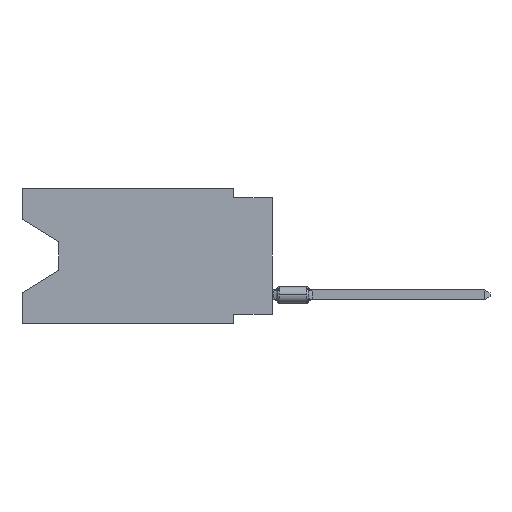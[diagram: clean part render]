
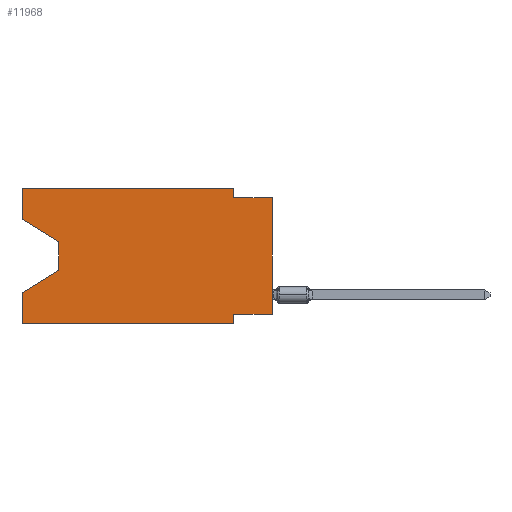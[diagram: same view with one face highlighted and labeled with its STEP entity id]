
A CAD part, left-side view. The second image highlights one B-rep face of the part: STEP entity #11968.
In plain terms, the highlighted planar face has unit normal (-1, 0, 0).
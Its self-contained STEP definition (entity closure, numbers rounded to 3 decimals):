
#106 = EDGE_CURVE ( 'NONE', #3288, #13067, #16867, .T. ) ;
#552 = CARTESIAN_POINT ( 'NONE',  ( 0., 2.54, 0. ) ) ;
#591 = DIRECTION ( 'NONE',  ( 0., 1., 0. ) ) ;
#726 = VECTOR ( 'NONE', #15065, 1000. ) ;
#868 = VECTOR ( 'NONE', #11107, 1000. ) ;
#931 = VECTOR ( 'NONE', #11445, 1000. ) ;
#1129 = CARTESIAN_POINT ( 'NONE',  ( 0., 16.383, -2.038 ) ) ;
#1162 = ORIENTED_EDGE ( 'NONE', *, *, #19828, .T. ) ;
#1165 = VERTEX_POINT ( 'NONE', #9282 ) ;
#1702 = VECTOR ( 'NONE', #10590, 1000. ) ;
#1963 = CARTESIAN_POINT ( 'NONE',  ( 0., 0., -0.635 ) ) ;
#2157 = VERTEX_POINT ( 'NONE', #18144 ) ;
#2304 = CARTESIAN_POINT ( 'NONE',  ( 0., 0., -8.255 ) ) ;
#2683 = VERTEX_POINT ( 'NONE', #5898 ) ;
#2824 = ORIENTED_EDGE ( 'NONE', *, *, #8476, .T. ) ;
#3091 = CARTESIAN_POINT ( 'NONE',  ( 0., 2.54, 0. ) ) ;
#3111 = PLANE ( 'NONE',  #18982 ) ;
#3288 = VERTEX_POINT ( 'NONE', #23810 ) ;
#3625 = CARTESIAN_POINT ( 'NONE',  ( 0., 0., -0.635 ) ) ;
#3835 = VECTOR ( 'NONE', #10383, 1000. ) ;
#3993 = VERTEX_POINT ( 'NONE', #21806 ) ;
#4361 = CARTESIAN_POINT ( 'NONE',  ( 0., 16.383, -8.89 ) ) ;
#5076 = DIRECTION ( 'NONE',  ( 1., 0., 0. ) ) ;
#5306 = EDGE_CURVE ( 'NONE', #2157, #2683, #7173, .T. ) ;
#5634 = ORIENTED_EDGE ( 'NONE', *, *, #13589, .F. ) ;
#5898 = CARTESIAN_POINT ( 'NONE',  ( 0., 2.54, -8.89 ) ) ;
#6046 = CARTESIAN_POINT ( 'NONE',  ( 0., 16.383, -2.038 ) ) ;
#6144 = EDGE_LOOP ( 'NONE', ( #1162, #20517, #16473, #9289, #6242, #10947, #17091, #2824, #5634, #23249, #10816, #18569 ) ) ;
#6242 = ORIENTED_EDGE ( 'NONE', *, *, #17470, .T. ) ;
#6563 = CARTESIAN_POINT ( 'NONE',  ( 0., 16.383, 0. ) ) ;
#6565 = EDGE_CURVE ( 'NONE', #3993, #3288, #13773, .T. ) ;
#6923 = CARTESIAN_POINT ( 'NONE',  ( 0., 16.383, 0. ) ) ;
#6986 = EDGE_CURVE ( 'NONE', #16297, #1165, #12475, .T. ) ;
#7022 = LINE ( 'NONE', #12564, #1702 ) ;
#7173 = LINE ( 'NONE', #12837, #11865 ) ;
#7303 = VERTEX_POINT ( 'NONE', #22535 ) ;
#7322 = LINE ( 'NONE', #13110, #726 ) ;
#7744 = LINE ( 'NONE', #1963, #931 ) ;
#8208 = EDGE_CURVE ( 'NONE', #11666, #19872, #11739, .T. ) ;
#8476 = EDGE_CURVE ( 'NONE', #7303, #21002, #22764, .T. ) ;
#9282 = CARTESIAN_POINT ( 'NONE',  ( 0., 16.383, 0. ) ) ;
#9289 = ORIENTED_EDGE ( 'NONE', *, *, #12259, .F. ) ;
#9373 = VERTEX_POINT ( 'NONE', #4361 ) ;
#10278 = EDGE_CURVE ( 'NONE', #7303, #2157, #11542, .T. ) ;
#10383 = DIRECTION ( 'NONE',  ( 0., 0., 1. ) ) ;
#10486 = LINE ( 'NONE', #1129, #12866 ) ;
#10590 = DIRECTION ( 'NONE',  ( 0., 0., 1. ) ) ;
#10816 = ORIENTED_EDGE ( 'NONE', *, *, #16095, .F. ) ;
#10947 = ORIENTED_EDGE ( 'NONE', *, *, #5306, .F. ) ;
#11107 = DIRECTION ( 'NONE',  ( 0., 0., 1. ) ) ;
#11354 = DIRECTION ( 'NONE',  ( 0., 0., -1. ) ) ;
#11445 = DIRECTION ( 'NONE',  ( 0., -1., 0. ) ) ;
#11542 = LINE ( 'NONE', #2304, #17362 ) ;
#11579 = CARTESIAN_POINT ( 'NONE',  ( 0., 13.97, -5.385 ) ) ;
#11666 = VERTEX_POINT ( 'NONE', #3091 ) ;
#11739 = LINE ( 'NONE', #552, #18933 ) ;
#11865 = VECTOR ( 'NONE', #11354, 1000. ) ;
#11869 = DIRECTION ( 'NONE',  ( 0., 0., -1. ) ) ;
#11968 = ADVANCED_FACE ( 'NONE', ( #21800 ), #3111, .F. ) ;
#12259 = EDGE_CURVE ( 'NONE', #9373, #13067, #7022, .T. ) ;
#12470 = LINE ( 'NONE', #19954, #19007 ) ;
#12475 = LINE ( 'NONE', #6563, #3835 ) ;
#12564 = CARTESIAN_POINT ( 'NONE',  ( 0., 16.383, 0. ) ) ;
#12837 = CARTESIAN_POINT ( 'NONE',  ( 0., 2.54, -8.89 ) ) ;
#12866 = VECTOR ( 'NONE', #16147, 1000. ) ;
#13067 = VERTEX_POINT ( 'NONE', #16391 ) ;
#13110 = CARTESIAN_POINT ( 'NONE',  ( 0., 16.383, -8.89 ) ) ;
#13176 = DIRECTION ( 'NONE',  ( 0., 0.855, -0.519 ) ) ;
#13589 = EDGE_CURVE ( 'NONE', #19872, #21002, #7744, .T. ) ;
#13643 = VECTOR ( 'NONE', #21386, 1000. ) ;
#13773 = LINE ( 'NONE', #23234, #13643 ) ;
#15065 = DIRECTION ( 'NONE',  ( 0., -1., 0. ) ) ;
#16095 = EDGE_CURVE ( 'NONE', #1165, #11666, #12470, .T. ) ;
#16147 = DIRECTION ( 'NONE',  ( 0., -0.855, -0.519 ) ) ;
#16297 = VERTEX_POINT ( 'NONE', #6046 ) ;
#16391 = CARTESIAN_POINT ( 'NONE',  ( 0., 16.383, -6.852 ) ) ;
#16473 = ORIENTED_EDGE ( 'NONE', *, *, #106, .T. ) ;
#16867 = LINE ( 'NONE', #11579, #24119 ) ;
#17091 = ORIENTED_EDGE ( 'NONE', *, *, #10278, .F. ) ;
#17362 = VECTOR ( 'NONE', #591, 1000. ) ;
#17470 = EDGE_CURVE ( 'NONE', #9373, #2683, #7322, .T. ) ;
#18144 = CARTESIAN_POINT ( 'NONE',  ( 0., 2.54, -8.255 ) ) ;
#18569 = ORIENTED_EDGE ( 'NONE', *, *, #6986, .F. ) ;
#18933 = VECTOR ( 'NONE', #11869, 1000. ) ;
#18982 = AXIS2_PLACEMENT_3D ( 'NONE', #6923, #5076, #21920 ) ;
#19007 = VECTOR ( 'NONE', #19834, 1000. ) ;
#19828 = EDGE_CURVE ( 'NONE', #16297, #3993, #10486, .T. ) ;
#19834 = DIRECTION ( 'NONE',  ( 0., -1., 0. ) ) ;
#19872 = VERTEX_POINT ( 'NONE', #20672 ) ;
#19954 = CARTESIAN_POINT ( 'NONE',  ( 0., 16.383, 0. ) ) ;
#20430 = CARTESIAN_POINT ( 'NONE',  ( 0., 0., 0. ) ) ;
#20517 = ORIENTED_EDGE ( 'NONE', *, *, #6565, .T. ) ;
#20672 = CARTESIAN_POINT ( 'NONE',  ( 0., 2.54, -0.635 ) ) ;
#21002 = VERTEX_POINT ( 'NONE', #3625 ) ;
#21386 = DIRECTION ( 'NONE',  ( 0., 0., -1. ) ) ;
#21800 = FACE_OUTER_BOUND ( 'NONE', #6144, .T. ) ;
#21806 = CARTESIAN_POINT ( 'NONE',  ( 0., 13.97, -3.505 ) ) ;
#21920 = DIRECTION ( 'NONE',  ( 0., 0., -1. ) ) ;
#22535 = CARTESIAN_POINT ( 'NONE',  ( 0., 0., -8.255 ) ) ;
#22764 = LINE ( 'NONE', #20430, #868 ) ;
#23234 = CARTESIAN_POINT ( 'NONE',  ( 0., 13.97, -3.505 ) ) ;
#23249 = ORIENTED_EDGE ( 'NONE', *, *, #8208, .F. ) ;
#23810 = CARTESIAN_POINT ( 'NONE',  ( 0., 13.97, -5.385 ) ) ;
#24119 = VECTOR ( 'NONE', #13176, 1000. ) ;
